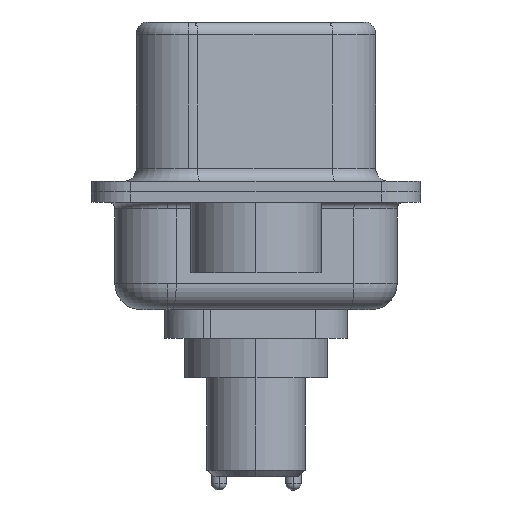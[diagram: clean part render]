
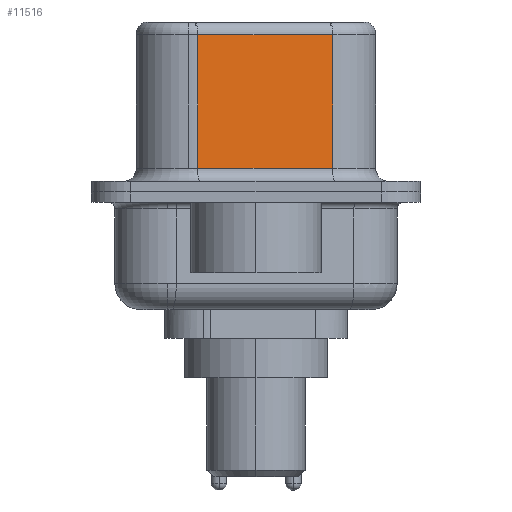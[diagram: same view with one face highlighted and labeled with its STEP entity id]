
A CAD part, left-side view. The second image highlights one B-rep face of the part: STEP entity #11516.
In plain terms, the highlighted planar face has unit normal (-0.985, -0.174, 0).
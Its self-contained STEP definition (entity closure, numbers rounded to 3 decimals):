
#71 = LINE ( 'NONE', #2087, #15154 ) ;
#319 = DIRECTION ( 'NONE',  ( 0., 0., -1. ) ) ;
#573 = ORIENTED_EDGE ( 'NONE', *, *, #22088, .T. ) ;
#2069 = ORIENTED_EDGE ( 'NONE', *, *, #11023, .T. ) ;
#2087 = CARTESIAN_POINT ( 'NONE',  ( 3.67, 2.233, 6.52 ) ) ;
#2593 = LINE ( 'NONE', #8362, #21690 ) ;
#2776 = LINE ( 'NONE', #14014, #7798 ) ;
#3223 = PLANE ( 'NONE',  #4418 ) ;
#4418 = AXIS2_PLACEMENT_3D ( 'NONE', #18095, #21721, #10779 ) ;
#5648 = CARTESIAN_POINT ( 'NONE',  ( 3.67, 2.233, 6.02 ) ) ;
#6587 = EDGE_CURVE ( 'NONE', #7132, #9850, #71, .T. ) ;
#6651 = CARTESIAN_POINT ( 'NONE',  ( 3.67, 2.233, 0.9 ) ) ;
#7132 = VERTEX_POINT ( 'NONE', #5648 ) ;
#7798 = VECTOR ( 'NONE', #23099, 1000. ) ;
#8362 = CARTESIAN_POINT ( 'NONE',  ( 4.58, -2.927, 6.02 ) ) ;
#8873 = FACE_OUTER_BOUND ( 'NONE', #21790, .T. ) ;
#9850 = VERTEX_POINT ( 'NONE', #6651 ) ;
#10779 = DIRECTION ( 'NONE',  ( -0.174, 0.985, 0. ) ) ;
#11023 = EDGE_CURVE ( 'NONE', #9850, #20146, #17024, .T. ) ;
#11516 = ADVANCED_FACE ( 'NONE', ( #8873 ), #3223, .F. ) ;
#12136 = VECTOR ( 'NONE', #18756, 1000. ) ;
#13256 = CARTESIAN_POINT ( 'NONE',  ( 4.58, -2.927, 0.9 ) ) ;
#14014 = CARTESIAN_POINT ( 'NONE',  ( 4.58, -2.927, 6.52 ) ) ;
#15154 = VECTOR ( 'NONE', #319, 1000. ) ;
#15707 = CARTESIAN_POINT ( 'NONE',  ( 4.58, -2.927, 0.9 ) ) ;
#16027 = ORIENTED_EDGE ( 'NONE', *, *, #16783, .F. ) ;
#16584 = ORIENTED_EDGE ( 'NONE', *, *, #6587, .T. ) ;
#16783 = EDGE_CURVE ( 'NONE', #16971, #20146, #2776, .T. ) ;
#16971 = VERTEX_POINT ( 'NONE', #19872 ) ;
#17024 = LINE ( 'NONE', #13256, #12136 ) ;
#18095 = CARTESIAN_POINT ( 'NONE',  ( 4.58, -2.927, 6.52 ) ) ;
#18756 = DIRECTION ( 'NONE',  ( 0.174, -0.985, 0. ) ) ;
#19872 = CARTESIAN_POINT ( 'NONE',  ( 4.58, -2.927, 6.02 ) ) ;
#20146 = VERTEX_POINT ( 'NONE', #15707 ) ;
#21191 = DIRECTION ( 'NONE',  ( -0.174, 0.985, 0. ) ) ;
#21690 = VECTOR ( 'NONE', #21191, 1000. ) ;
#21721 = DIRECTION ( 'NONE',  ( 0.985, 0.174, 0. ) ) ;
#21790 = EDGE_LOOP ( 'NONE', ( #16027, #573, #16584, #2069 ) ) ;
#22088 = EDGE_CURVE ( 'NONE', #16971, #7132, #2593, .T. ) ;
#23099 = DIRECTION ( 'NONE',  ( 0., 0., -1. ) ) ;
